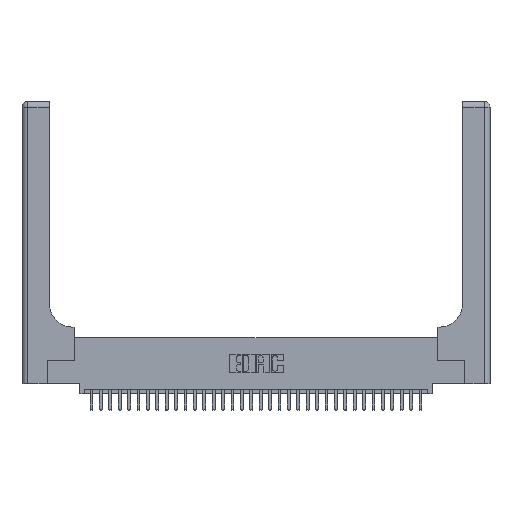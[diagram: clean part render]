
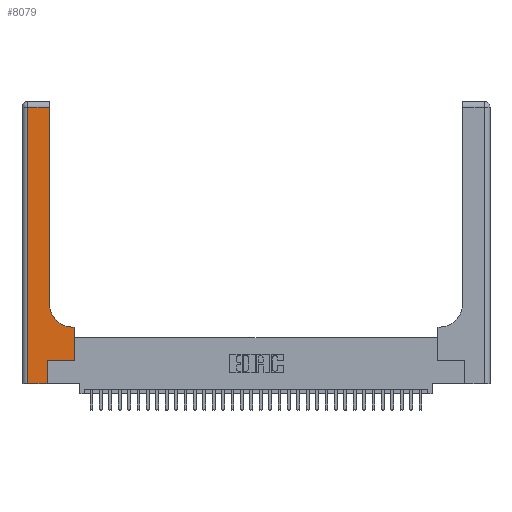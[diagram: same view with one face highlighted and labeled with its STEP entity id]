
A CAD part, top view. The second image highlights one B-rep face of the part: STEP entity #8079.
In plain terms, the highlighted planar face has unit normal (0, 0, 1).
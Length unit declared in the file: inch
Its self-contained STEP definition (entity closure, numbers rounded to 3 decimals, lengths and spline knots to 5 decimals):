
#39 = ORIENTED_EDGE ( 'NONE', *, *, #32679, .T. ) ;
#1255 = CIRCLE ( 'NONE', #6533, 0.25 ) ;
#1263 = CARTESIAN_POINT ( 'NONE',  ( 0.269, 0., 0.37 ) ) ;
#1424 = VERTEX_POINT ( 'NONE', #3017 ) ;
#1523 = EDGE_CURVE ( 'NONE', #32611, #27737, #4486, .T. ) ;
#1906 = CARTESIAN_POINT ( 'NONE',  ( 0.2915, 0.85, 0.37 ) ) ;
#2622 = VECTOR ( 'NONE', #27236, 39.37008 ) ;
#3017 = CARTESIAN_POINT ( 'NONE',  ( 0.5585, 0.6, 0.37 ) ) ;
#3216 = AXIS2_PLACEMENT_3D ( 'NONE', #29065, #31658, #34249 ) ;
#3303 = CARTESIAN_POINT ( 'NONE',  ( 0.2915, 3., 0.37 ) ) ;
#3439 = EDGE_CURVE ( 'NONE', #1424, #18166, #13973, .T. ) ;
#3981 = VECTOR ( 'NONE', #31507, 39.37008 ) ;
#4486 = LINE ( 'NONE', #32115, #9926 ) ;
#4496 = EDGE_CURVE ( 'NONE', #27438, #1424, #27171, .T. ) ;
#4654 = LINE ( 'NONE', #14233, #30417 ) ;
#5066 = CARTESIAN_POINT ( 'NONE',  ( 0.5415, 0.85, 0.37 ) ) ;
#6205 = VECTOR ( 'NONE', #18666, 39.37008 ) ;
#6533 = AXIS2_PLACEMENT_3D ( 'NONE', #5066, #7881, #31961 ) ;
#6782 = CARTESIAN_POINT ( 'NONE',  ( 0.5415, 0.6, 0.37 ) ) ;
#7132 = LINE ( 'NONE', #20208, #29170 ) ;
#7748 = VERTEX_POINT ( 'NONE', #12124 ) ;
#7881 = DIRECTION ( 'NONE',  ( 0., 0., -1. ) ) ;
#8079 = ADVANCED_FACE ( 'NONE', ( #12436 ), #23456, .F. ) ;
#8545 = CARTESIAN_POINT ( 'NONE',  ( 0.5585, 0.25, 0.37 ) ) ;
#8842 = CARTESIAN_POINT ( 'NONE',  ( 0.269, 0.25, 0.37 ) ) ;
#9003 = ORIENTED_EDGE ( 'NONE', *, *, #1523, .T. ) ;
#9485 = ORIENTED_EDGE ( 'NONE', *, *, #31674, .T. ) ;
#9737 = LINE ( 'NONE', #3303, #2622 ) ;
#9926 = VECTOR ( 'NONE', #27393, 39.37008 ) ;
#10638 = CARTESIAN_POINT ( 'NONE',  ( 0.06, 3., 0.37 ) ) ;
#10795 = VERTEX_POINT ( 'NONE', #30872 ) ;
#11641 = ORIENTED_EDGE ( 'NONE', *, *, #20678, .T. ) ;
#11846 = DIRECTION ( 'NONE',  ( 0., 1., 0. ) ) ;
#12124 = CARTESIAN_POINT ( 'NONE',  ( 0.06, 0., 0.37 ) ) ;
#12436 = FACE_OUTER_BOUND ( 'NONE', #18510, .T. ) ;
#12565 = ORIENTED_EDGE ( 'NONE', *, *, #4496, .T. ) ;
#12935 = VERTEX_POINT ( 'NONE', #8842 ) ;
#13168 = ORIENTED_EDGE ( 'NONE', *, *, #3439, .T. ) ;
#13973 = LINE ( 'NONE', #15594, #3981 ) ;
#14233 = CARTESIAN_POINT ( 'NONE',  ( 0., 0., 0.37 ) ) ;
#14742 = CARTESIAN_POINT ( 'NONE',  ( 0.5585, 0.25, 0.37 ) ) ;
#14892 = DIRECTION ( 'NONE',  ( 1., 0., 0. ) ) ;
#15279 = EDGE_CURVE ( 'NONE', #12935, #27438, #7132, .T. ) ;
#15594 = CARTESIAN_POINT ( 'NONE',  ( 0.2915, 0.6, 0.37 ) ) ;
#15673 = ORIENTED_EDGE ( 'NONE', *, *, #15279, .T. ) ;
#15761 = DIRECTION ( 'NONE',  ( 0., 1., 0. ) ) ;
#17356 = CARTESIAN_POINT ( 'NONE',  ( 0.2915, 2.94, 0.37 ) ) ;
#17810 = VERTEX_POINT ( 'NONE', #1906 ) ;
#18166 = VERTEX_POINT ( 'NONE', #6782 ) ;
#18510 = EDGE_LOOP ( 'NONE', ( #20009, #9003, #9485, #34295, #39, #15673, #12565, #13168, #11641 ) ) ;
#18666 = DIRECTION ( 'NONE',  ( 0., -1., 0. ) ) ;
#18904 = EDGE_CURVE ( 'NONE', #7748, #10795, #4654, .T. ) ;
#19506 = VECTOR ( 'NONE', #11846, 39.37008 ) ;
#20009 = ORIENTED_EDGE ( 'NONE', *, *, #29925, .T. ) ;
#20155 = VECTOR ( 'NONE', #15761, 39.37008 ) ;
#20208 = CARTESIAN_POINT ( 'NONE',  ( 0.269, 0.25, 0.37 ) ) ;
#20376 = LINE ( 'NONE', #1263, #19506 ) ;
#20678 = EDGE_CURVE ( 'NONE', #18166, #17810, #1255, .T. ) ;
#23456 = PLANE ( 'NONE',  #3216 ) ;
#25182 = CARTESIAN_POINT ( 'NONE',  ( 0.06, 2.94, 0.37 ) ) ;
#26602 = LINE ( 'NONE', #10638, #6205 ) ;
#27171 = LINE ( 'NONE', #8545, #20155 ) ;
#27236 = DIRECTION ( 'NONE',  ( 0., 1., 0. ) ) ;
#27393 = DIRECTION ( 'NONE',  ( -1., 0., 0. ) ) ;
#27438 = VERTEX_POINT ( 'NONE', #14742 ) ;
#27737 = VERTEX_POINT ( 'NONE', #25182 ) ;
#29065 = CARTESIAN_POINT ( 'NONE',  ( 0., 3., 0.37 ) ) ;
#29170 = VECTOR ( 'NONE', #14892, 39.37008 ) ;
#29925 = EDGE_CURVE ( 'NONE', #17810, #32611, #9737, .T. ) ;
#30417 = VECTOR ( 'NONE', #33917, 39.37008 ) ;
#30872 = CARTESIAN_POINT ( 'NONE',  ( 0.269, 0., 0.37 ) ) ;
#31507 = DIRECTION ( 'NONE',  ( -1., 0., 0. ) ) ;
#31658 = DIRECTION ( 'NONE',  ( 0., 0., -1. ) ) ;
#31674 = EDGE_CURVE ( 'NONE', #27737, #7748, #26602, .T. ) ;
#31961 = DIRECTION ( 'NONE',  ( 1., 0., 0. ) ) ;
#32115 = CARTESIAN_POINT ( 'NONE',  ( 0., 2.94, 0.37 ) ) ;
#32611 = VERTEX_POINT ( 'NONE', #17356 ) ;
#32679 = EDGE_CURVE ( 'NONE', #10795, #12935, #20376, .T. ) ;
#33917 = DIRECTION ( 'NONE',  ( 1., 0., 0. ) ) ;
#34249 = DIRECTION ( 'NONE',  ( -1., 0., 0. ) ) ;
#34295 = ORIENTED_EDGE ( 'NONE', *, *, #18904, .T. ) ;
